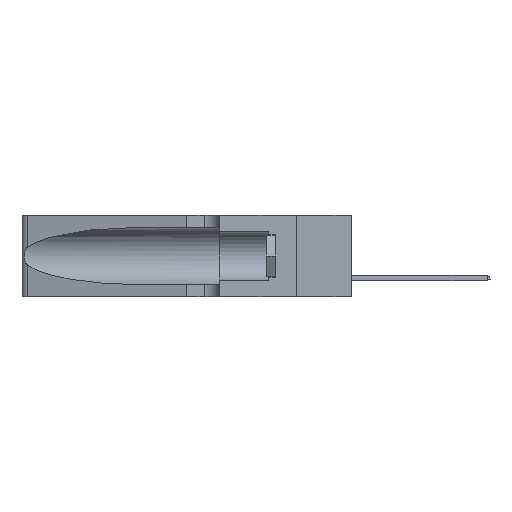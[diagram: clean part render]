
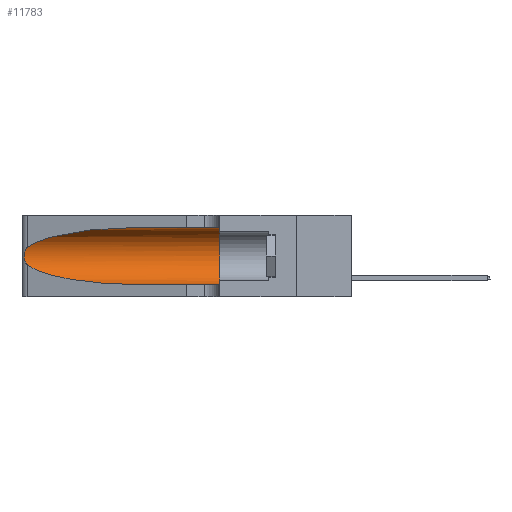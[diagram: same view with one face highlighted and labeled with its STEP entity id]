
A CAD part, left-side view. The second image highlights one B-rep face of the part: STEP entity #11783.
In plain terms, the highlighted cylindrical face has radius 3.308 mm (diameter 6.617 mm), a partial arc.
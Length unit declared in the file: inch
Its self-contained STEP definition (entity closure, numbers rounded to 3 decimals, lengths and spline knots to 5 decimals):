
#180 = DIRECTION ( 'NONE',  ( 0., 0., -1. ) ) ;
#284 = LINE ( 'NONE', #5104, #9677 ) ;
#302 = CARTESIAN_POINT ( 'NONE',  ( 0.26075, 1.23896, 0.178 ) ) ;
#471 = CARTESIAN_POINT ( 'NONE',  ( 0.25639, 1.23186, 0.15144 ) ) ;
#492 = DIRECTION ( 'NONE',  ( 0., 1., 0. ) ) ;
#566 = VERTEX_POINT ( 'NONE', #4568 ) ;
#1475 = EDGE_CURVE ( 'NONE', #12721, #5995, #12297, .T. ) ;
#2076 = ORIENTED_EDGE ( 'NONE', *, *, #22051, .T. ) ;
#2598 =( BOUNDED_CURVE ( )  B_SPLINE_CURVE ( 3, ( #5272, #5661, #21084, #9213 ),
 .UNSPECIFIED., .F., .T. ) 
 B_SPLINE_CURVE_WITH_KNOTS ( ( 4, 4 ),
 ( 1.5708, 2.84003 ),
 .UNSPECIFIED. ) 
 CURVE ( )  GEOMETRIC_REPRESENTATION_ITEM ( )  RATIONAL_B_SPLINE_CURVE ( ( 1., 0.87, 0.87, 1. ) ) 
 REPRESENTATION_ITEM ( '' )  );
#2824 = CARTESIAN_POINT ( 'NONE',  ( 0.18966, 0.96281, 0.05475 ) ) ;
#3189 = LINE ( 'NONE', #13912, #14688 ) ;
#3218 = CARTESIAN_POINT ( 'NONE',  ( 0.1305, 0.35, 0.05475 ) ) ;
#3262 = CARTESIAN_POINT ( 'NONE',  ( 0.25555, 1.22994, 0.2215 ) ) ;
#3732 = CARTESIAN_POINT ( 'NONE',  ( 0.25555, 1.22993, 0.14849 ) ) ;
#3951 = CARTESIAN_POINT ( 'NONE',  ( 0.25487, 1.22718, 0.14631 ) ) ;
#4047 = DIRECTION ( 'NONE',  ( 0., 0., 1. ) ) ;
#4208 = CARTESIAN_POINT ( 'NONE',  ( 0.1305, 0.35, 0.185 ) ) ;
#4568 = CARTESIAN_POINT ( 'NONE',  ( 0.25487, 1.22718, 0.14631 ) ) ;
#4777 = ORIENTED_EDGE ( 'NONE', *, *, #20222, .F. ) ;
#5104 = CARTESIAN_POINT ( 'NONE',  ( 0.1305, 1.61858, 0.05475 ) ) ;
#5124 = CARTESIAN_POINT ( 'NONE',  ( 0.1305, 0.72297, 0.31525 ) ) ;
#5272 = CARTESIAN_POINT ( 'NONE',  ( 0.1305, 0.72297, 0.31525 ) ) ;
#5300 = CYLINDRICAL_SURFACE ( 'NONE', #18031, 0.13025 ) ;
#5661 = CARTESIAN_POINT ( 'NONE',  ( 0.18966, 0.96281, 0.31525 ) ) ;
#5995 = VERTEX_POINT ( 'NONE', #3218 ) ;
#6531 = CARTESIAN_POINT ( 'NONE',  ( 0.25639, 1.23184, 0.21858 ) ) ;
#6836 = CARTESIAN_POINT ( 'NONE',  ( 0.25787, 1.23484, 0.2124 ) ) ;
#7148 = CARTESIAN_POINT ( 'NONE',  ( 0.25487, 1.22718, 0.22369 ) ) ;
#7195 = EDGE_CURVE ( 'NONE', #566, #7484, #15418, .T. ) ;
#7484 = VERTEX_POINT ( 'NONE', #13530 ) ;
#8041 = B_SPLINE_CURVE_WITH_KNOTS ( 'NONE', 3,
 ( #16769, #3262, #6531, #6836, #19044, #8644, #12711, #302, #10978, #12559, #12625, #471, #3732, #3951 ),
 .UNSPECIFIED., .F., .F.,
 ( 4, 2, 2, 2, 2, 2, 4 ),
 ( 0., 0.00027, 0.00053, 0.00107, 0.0016, 0.00187, 0.00214 ),
 .UNSPECIFIED. ) ;
#8644 = CARTESIAN_POINT ( 'NONE',  ( 0.26018, 1.23835, 0.19895 ) ) ;
#9213 = CARTESIAN_POINT ( 'NONE',  ( 0.25487, 1.22718, 0.22369 ) ) ;
#9516 = EDGE_LOOP ( 'NONE', ( #2076, #20425, #17593, #11889, #11089, #4777 ) ) ;
#9677 = VECTOR ( 'NONE', #17510, 39.37008 ) ;
#10894 = VERTEX_POINT ( 'NONE', #7148 ) ;
#10978 = CARTESIAN_POINT ( 'NONE',  ( 0.26017, 1.23833, 0.17102 ) ) ;
#11089 = ORIENTED_EDGE ( 'NONE', *, *, #1475, .F. ) ;
#11783 = ADVANCED_FACE ( 'NONE', ( #15679 ), #5300, .F. ) ;
#11889 = ORIENTED_EDGE ( 'NONE', *, *, #22463, .T. ) ;
#12297 = CIRCLE ( 'NONE', #15827, 0.13025 ) ;
#12559 = CARTESIAN_POINT ( 'NONE',  ( 0.25856, 1.23593, 0.16098 ) ) ;
#12625 = CARTESIAN_POINT ( 'NONE',  ( 0.25789, 1.23486, 0.15765 ) ) ;
#12711 = CARTESIAN_POINT ( 'NONE',  ( 0.26075, 1.23896, 0.19203 ) ) ;
#12721 = VERTEX_POINT ( 'NONE', #21659 ) ;
#13530 = CARTESIAN_POINT ( 'NONE',  ( 0.1305, 0.72297, 0.05475 ) ) ;
#13912 = CARTESIAN_POINT ( 'NONE',  ( 0.1305, 1.61858, 0.31525 ) ) ;
#14571 = CARTESIAN_POINT ( 'NONE',  ( 0.1305, 0.72297, 0.05475 ) ) ;
#14688 = VECTOR ( 'NONE', #19238, 39.37008 ) ;
#14704 = VERTEX_POINT ( 'NONE', #5124 ) ;
#14948 = EDGE_CURVE ( 'NONE', #10894, #566, #8041, .T. ) ;
#15418 =( BOUNDED_CURVE ( )  B_SPLINE_CURVE ( 3, ( #22083, #20428, #2824, #14571 ),
 .UNSPECIFIED., .F., .F. ) 
 B_SPLINE_CURVE_WITH_KNOTS ( ( 4, 4 ),
 ( 3.44316, 4.71239 ),
 .UNSPECIFIED. ) 
 CURVE ( )  GEOMETRIC_REPRESENTATION_ITEM ( )  RATIONAL_B_SPLINE_CURVE ( ( 1., 0.87, 0.87, 1. ) ) 
 REPRESENTATION_ITEM ( '' )  );
#15679 = FACE_OUTER_BOUND ( 'NONE', #9516, .T. ) ;
#15827 = AXIS2_PLACEMENT_3D ( 'NONE', #4208, #492, #4047 ) ;
#16769 = CARTESIAN_POINT ( 'NONE',  ( 0.25487, 1.22718, 0.22369 ) ) ;
#17510 = DIRECTION ( 'NONE',  ( 0., -1., 0. ) ) ;
#17593 = ORIENTED_EDGE ( 'NONE', *, *, #7195, .T. ) ;
#18031 = AXIS2_PLACEMENT_3D ( 'NONE', #19522, #21394, #180 ) ;
#19044 = CARTESIAN_POINT ( 'NONE',  ( 0.25854, 1.2359, 0.20912 ) ) ;
#19238 = DIRECTION ( 'NONE',  ( 0., -1., 0. ) ) ;
#19522 = CARTESIAN_POINT ( 'NONE',  ( 0.1305, 1.61858, 0.185 ) ) ;
#20222 = EDGE_CURVE ( 'NONE', #14704, #12721, #3189, .T. ) ;
#20425 = ORIENTED_EDGE ( 'NONE', *, *, #14948, .T. ) ;
#20428 = CARTESIAN_POINT ( 'NONE',  ( 0.2373, 1.15595, 0.08982 ) ) ;
#21084 = CARTESIAN_POINT ( 'NONE',  ( 0.2373, 1.15595, 0.28018 ) ) ;
#21394 = DIRECTION ( 'NONE',  ( 0., -1., 0. ) ) ;
#21659 = CARTESIAN_POINT ( 'NONE',  ( 0.1305, 0.35, 0.31525 ) ) ;
#22051 = EDGE_CURVE ( 'NONE', #14704, #10894, #2598, .T. ) ;
#22083 = CARTESIAN_POINT ( 'NONE',  ( 0.25487, 1.22718, 0.14631 ) ) ;
#22463 = EDGE_CURVE ( 'NONE', #7484, #5995, #284, .T. ) ;
